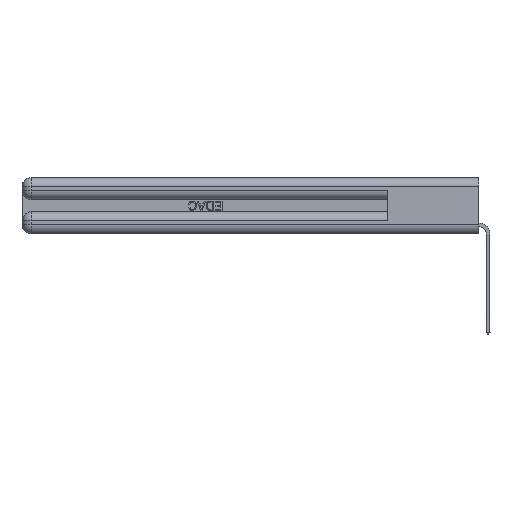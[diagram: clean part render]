
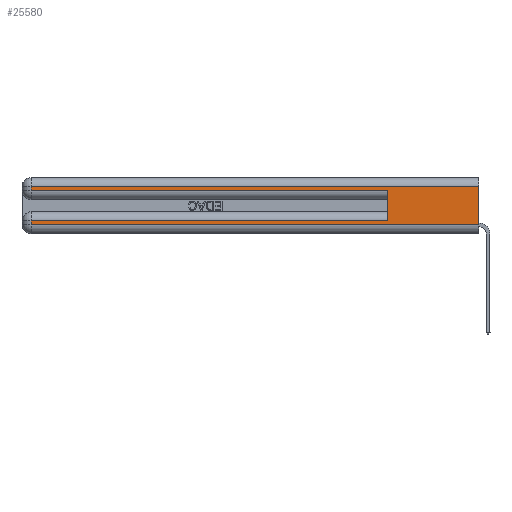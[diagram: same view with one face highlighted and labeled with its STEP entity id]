
A CAD part, left-side view. The second image highlights one B-rep face of the part: STEP entity #25580.
In plain terms, the highlighted planar face has unit normal (-1, 0, 0).
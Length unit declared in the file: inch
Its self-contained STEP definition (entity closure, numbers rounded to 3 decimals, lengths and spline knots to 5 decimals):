
#206 = VECTOR ( 'NONE', #30912, 39.37008 ) ;
#404 = EDGE_LOOP ( 'NONE', ( #12421, #30509, #31135, #25875, #4641, #4826, #15958, #19549 ) ) ;
#1082 = VECTOR ( 'NONE', #4531, 39.37008 ) ;
#1654 = VERTEX_POINT ( 'NONE', #20057 ) ;
#2587 = CARTESIAN_POINT ( 'NONE',  ( 0., 0.6, 0.085 ) ) ;
#3470 = VERTEX_POINT ( 'NONE', #2587 ) ;
#3814 = EDGE_CURVE ( 'NONE', #11494, #13972, #27954, .T. ) ;
#4531 = DIRECTION ( 'NONE',  ( 0., 0., -1. ) ) ;
#4641 = ORIENTED_EDGE ( 'NONE', *, *, #8890, .F. ) ;
#4826 = ORIENTED_EDGE ( 'NONE', *, *, #10753, .T. ) ;
#5885 = DIRECTION ( 'NONE',  ( 0., 0., 1. ) ) ;
#5947 = CARTESIAN_POINT ( 'NONE',  ( 0., 0., 0.31 ) ) ;
#6942 = LINE ( 'NONE', #16030, #206 ) ;
#8095 = CARTESIAN_POINT ( 'NONE',  ( 0., 0., 0.06 ) ) ;
#8890 = EDGE_CURVE ( 'NONE', #3470, #13972, #24387, .T. ) ;
#9015 = VECTOR ( 'NONE', #16679, 39.37008 ) ;
#9185 = CARTESIAN_POINT ( 'NONE',  ( 0., 0., 0.085 ) ) ;
#9711 = VECTOR ( 'NONE', #16558, 39.37008 ) ;
#9855 = DIRECTION ( 'NONE',  ( 1., 0., 0. ) ) ;
#10682 = VECTOR ( 'NONE', #11714, 39.37008 ) ;
#10753 = EDGE_CURVE ( 'NONE', #3470, #15816, #28826, .T. ) ;
#11286 = VECTOR ( 'NONE', #22178, 39.37008 ) ;
#11494 = VERTEX_POINT ( 'NONE', #29238 ) ;
#11598 = EDGE_CURVE ( 'NONE', #22595, #30832, #17896, .T. ) ;
#11714 = DIRECTION ( 'NONE',  ( 0., 0., -1. ) ) ;
#12087 = CARTESIAN_POINT ( 'NONE',  ( 0., 2.94, 0.37 ) ) ;
#12421 = ORIENTED_EDGE ( 'NONE', *, *, #11598, .F. ) ;
#12450 = EDGE_CURVE ( 'NONE', #22595, #24275, #6942, .T. ) ;
#13409 = CARTESIAN_POINT ( 'NONE',  ( 0., 0.6, 0.145 ) ) ;
#13972 = VERTEX_POINT ( 'NONE', #29226 ) ;
#14667 = CARTESIAN_POINT ( 'NONE',  ( 0., 0., 0.37 ) ) ;
#15816 = VERTEX_POINT ( 'NONE', #26710 ) ;
#15958 = ORIENTED_EDGE ( 'NONE', *, *, #24915, .T. ) ;
#16030 = CARTESIAN_POINT ( 'NONE',  ( 0., 0., 0.31 ) ) ;
#16558 = DIRECTION ( 'NONE',  ( 0., -1., 0. ) ) ;
#16679 = DIRECTION ( 'NONE',  ( 0., 1., 0. ) ) ;
#17896 = LINE ( 'NONE', #14667, #11286 ) ;
#19549 = ORIENTED_EDGE ( 'NONE', *, *, #31853, .T. ) ;
#19752 = PLANE ( 'NONE',  #31825 ) ;
#20057 = CARTESIAN_POINT ( 'NONE',  ( 0., 2.94, 0.06 ) ) ;
#20255 = LINE ( 'NONE', #12087, #1082 ) ;
#20608 = FACE_OUTER_BOUND ( 'NONE', #404, .T. ) ;
#21475 = CARTESIAN_POINT ( 'NONE',  ( 0., 0., 0.285 ) ) ;
#21527 = CARTESIAN_POINT ( 'NONE',  ( 0., 0., 0.06 ) ) ;
#22178 = DIRECTION ( 'NONE',  ( 0., 0., -1. ) ) ;
#22595 = VERTEX_POINT ( 'NONE', #5947 ) ;
#24073 = CARTESIAN_POINT ( 'NONE',  ( 0., 2.94, 0.37 ) ) ;
#24275 = VERTEX_POINT ( 'NONE', #29553 ) ;
#24387 = LINE ( 'NONE', #13409, #30231 ) ;
#24674 = LINE ( 'NONE', #24073, #10682 ) ;
#24710 = CARTESIAN_POINT ( 'NONE',  ( 0., 0., 0.37 ) ) ;
#24915 = EDGE_CURVE ( 'NONE', #15816, #1654, #20255, .T. ) ;
#24919 = VECTOR ( 'NONE', #30464, 39.37008 ) ;
#25580 = ADVANCED_FACE ( 'NONE', ( #20608 ), #19752, .F. ) ;
#25875 = ORIENTED_EDGE ( 'NONE', *, *, #3814, .T. ) ;
#26710 = CARTESIAN_POINT ( 'NONE',  ( 0., 2.94, 0.085 ) ) ;
#27216 = DIRECTION ( 'NONE',  ( 0., 0., -1. ) ) ;
#27954 = LINE ( 'NONE', #21475, #9711 ) ;
#28826 = LINE ( 'NONE', #9185, #9015 ) ;
#29226 = CARTESIAN_POINT ( 'NONE',  ( 0., 0.6, 0.285 ) ) ;
#29238 = CARTESIAN_POINT ( 'NONE',  ( 0., 2.94, 0.285 ) ) ;
#29553 = CARTESIAN_POINT ( 'NONE',  ( 0., 2.94, 0.31 ) ) ;
#29839 = EDGE_CURVE ( 'NONE', #24275, #11494, #24674, .T. ) ;
#29995 = LINE ( 'NONE', #8095, #24919 ) ;
#30231 = VECTOR ( 'NONE', #5885, 39.37008 ) ;
#30464 = DIRECTION ( 'NONE',  ( 0., -1., 0. ) ) ;
#30509 = ORIENTED_EDGE ( 'NONE', *, *, #12450, .T. ) ;
#30832 = VERTEX_POINT ( 'NONE', #21527 ) ;
#30912 = DIRECTION ( 'NONE',  ( 0., 1., 0. ) ) ;
#31135 = ORIENTED_EDGE ( 'NONE', *, *, #29839, .T. ) ;
#31825 = AXIS2_PLACEMENT_3D ( 'NONE', #24710, #9855, #27216 ) ;
#31853 = EDGE_CURVE ( 'NONE', #1654, #30832, #29995, .T. ) ;
